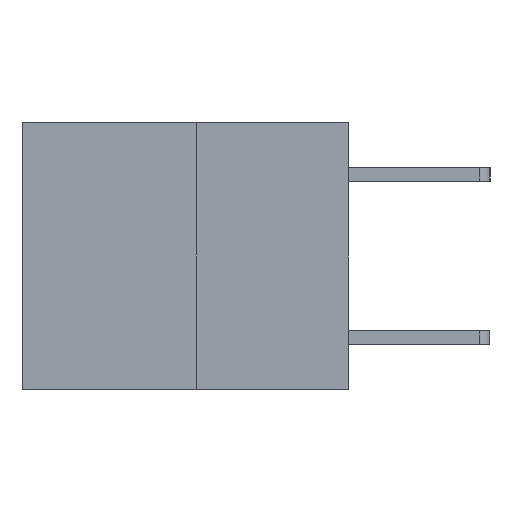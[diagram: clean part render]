
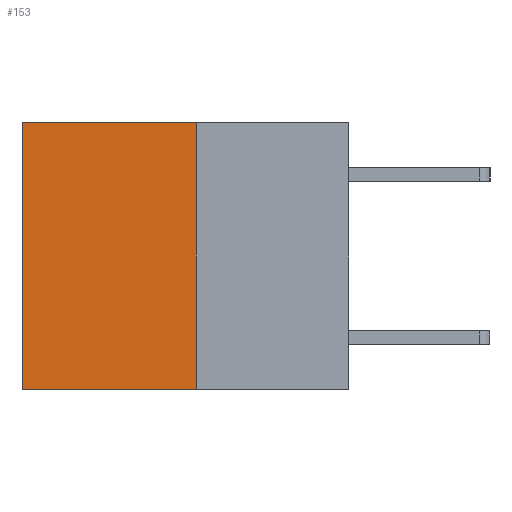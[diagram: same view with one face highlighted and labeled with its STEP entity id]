
A CAD part, left-side view. The second image highlights one B-rep face of the part: STEP entity #153.
In plain terms, the highlighted planar face has unit normal (-1, 0, 0).
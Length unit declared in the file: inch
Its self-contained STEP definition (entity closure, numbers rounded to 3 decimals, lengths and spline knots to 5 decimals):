
#153 = ADVANCED_FACE ( 'NONE', ( #3414 ), #3925, .F. ) ;
#299 = EDGE_CURVE ( 'NONE', #8991, #7299, #4708, .T. ) ;
#551 = EDGE_CURVE ( 'NONE', #9771, #7299, #4695, .T. ) ;
#647 = ORIENTED_EDGE ( 'NONE', *, *, #6746, .F. ) ;
#1244 = CARTESIAN_POINT ( 'NONE',  ( 0.3165, 0.28, -0.49 ) ) ;
#1542 = DIRECTION ( 'NONE',  ( 0., 0., -1. ) ) ;
#1872 = VERTEX_POINT ( 'NONE', #6553 ) ;
#2603 = CARTESIAN_POINT ( 'NONE',  ( 0.3165, 0.6, 0. ) ) ;
#3290 = CARTESIAN_POINT ( 'NONE',  ( 0.3165, 0.6, -0.49 ) ) ;
#3414 = FACE_OUTER_BOUND ( 'NONE', #6632, .T. ) ;
#3426 = DIRECTION ( 'NONE',  ( 0., 0., -1. ) ) ;
#3925 = PLANE ( 'NONE',  #7571 ) ;
#3999 = LINE ( 'NONE', #5809, #9078 ) ;
#4529 = ORIENTED_EDGE ( 'NONE', *, *, #299, .T. ) ;
#4573 = VECTOR ( 'NONE', #10475, 39.37008 ) ;
#4695 = LINE ( 'NONE', #5456, #4573 ) ;
#4708 = LINE ( 'NONE', #3290, #7250 ) ;
#4949 = ORIENTED_EDGE ( 'NONE', *, *, #551, .F. ) ;
#5456 = CARTESIAN_POINT ( 'NONE',  ( 0.3165, 0.28, -0.49 ) ) ;
#5809 = CARTESIAN_POINT ( 'NONE',  ( 0.3165, 0.28, -0.49 ) ) ;
#5863 = ORIENTED_EDGE ( 'NONE', *, *, #10729, .T. ) ;
#6376 = DIRECTION ( 'NONE',  ( 0., 0., -1. ) ) ;
#6553 = CARTESIAN_POINT ( 'NONE',  ( 0.3165, 0.28, 0. ) ) ;
#6591 = CARTESIAN_POINT ( 'NONE',  ( 0.3165, 0.6, -0.49 ) ) ;
#6620 = LINE ( 'NONE', #6789, #7294 ) ;
#6632 = EDGE_LOOP ( 'NONE', ( #4529, #4949, #647, #5863 ) ) ;
#6746 = EDGE_CURVE ( 'NONE', #1872, #9771, #3999, .T. ) ;
#6789 = CARTESIAN_POINT ( 'NONE',  ( 0.3165, 0.28, 0. ) ) ;
#7250 = VECTOR ( 'NONE', #1542, 39.37008 ) ;
#7294 = VECTOR ( 'NONE', #9522, 39.37008 ) ;
#7299 = VERTEX_POINT ( 'NONE', #6591 ) ;
#7571 = AXIS2_PLACEMENT_3D ( 'NONE', #1244, #10630, #6376 ) ;
#8991 = VERTEX_POINT ( 'NONE', #2603 ) ;
#9078 = VECTOR ( 'NONE', #3426, 39.37008 ) ;
#9522 = DIRECTION ( 'NONE',  ( 0., 1., 0. ) ) ;
#9656 = CARTESIAN_POINT ( 'NONE',  ( 0.3165, 0.28, -0.49 ) ) ;
#9771 = VERTEX_POINT ( 'NONE', #9656 ) ;
#10475 = DIRECTION ( 'NONE',  ( 0., 1., 0. ) ) ;
#10630 = DIRECTION ( 'NONE',  ( 1., 0., 0. ) ) ;
#10729 = EDGE_CURVE ( 'NONE', #1872, #8991, #6620, .T. ) ;
